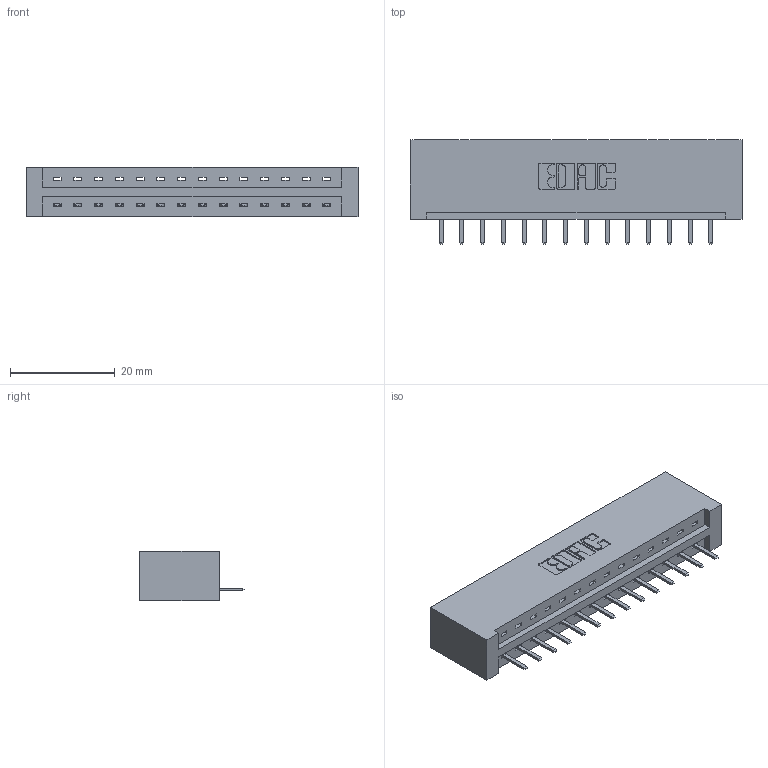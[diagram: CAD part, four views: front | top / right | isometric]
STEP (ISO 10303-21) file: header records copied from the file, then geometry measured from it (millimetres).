
FILE_DESCRIPTION (( 'STEP AP203' ), '1' );
FILE_NAME ('337-014-520-101.STEP', '2019-09-28T02:57:03', ( '' ), ( '' ), 'SwSTEP 2.0', 'SolidWorks 2016', '' );
FILE_SCHEMA (( 'CONFIG_CONTROL_DESIGN' ));
Length unit declared in the file: inch
Products named in the file (3): 345-292-001_345-293-120; 337-014-520-101; 337 Part_No Mounting Lugs
Assembly tree (15 placements, depth 2):
  337-014-520-101
    337 Part_No Mounting Lugs
    345-292-001_345-293-120  x14
Bounding box: 63.35 x 20.02 x 9.4 mm (x, y, z)
Volume: 6932 mm3; surface area: 6844.2 mm2
Topology: 15 solids, 15 shells, 1030 faces, 3031 edges, 1982 vertices
Faces by surface type: plane 738, cylinder 292
Entity records: 13865 total; most frequent: CARTESIAN_POINT 2432, ORIENTED_EDGE 2370, DIRECTION 2085, EDGE_CURVE 1185, LINE 1061, VECTOR 1061, VERTEX_POINT 786, AXIS2_PLACEMENT_3D 512
